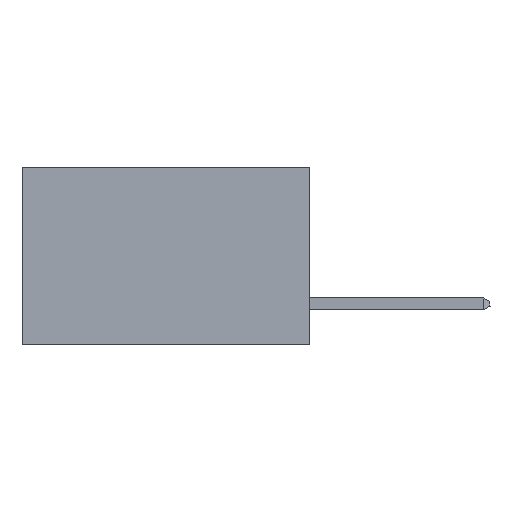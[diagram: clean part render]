
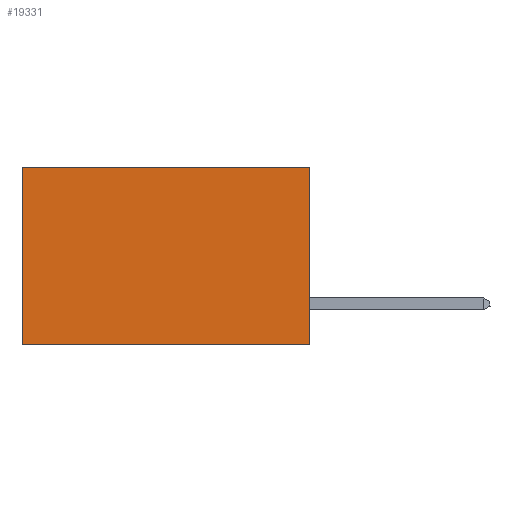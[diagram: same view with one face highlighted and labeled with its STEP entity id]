
A CAD part, left-side view. The second image highlights one B-rep face of the part: STEP entity #19331.
In plain terms, the highlighted planar face has unit normal (-1, 0, 0).
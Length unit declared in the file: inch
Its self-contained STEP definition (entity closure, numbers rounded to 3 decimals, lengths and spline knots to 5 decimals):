
#1119 = VERTEX_POINT ( 'NONE', #47202 ) ;
#1711 = CARTESIAN_POINT ( 'NONE',  ( 0.2875, 0., -0.37 ) ) ;
#5896 = AXIS2_PLACEMENT_3D ( 'NONE', #39786, #47557, #16915 ) ;
#8438 = EDGE_CURVE ( 'NONE', #30630, #1119, #39159, .T. ) ;
#9958 = CARTESIAN_POINT ( 'NONE',  ( 0.2875, 0.6, 0. ) ) ;
#10521 = EDGE_CURVE ( 'NONE', #29294, #42507, #29275, .T. ) ;
#12382 = DIRECTION ( 'NONE',  ( 0., 0., -1. ) ) ;
#14292 = CARTESIAN_POINT ( 'NONE',  ( 0.2875, 0., 0. ) ) ;
#16915 = DIRECTION ( 'NONE',  ( 0., 0., -1. ) ) ;
#17971 = VECTOR ( 'NONE', #47672, 39.37008 ) ;
#18190 = EDGE_CURVE ( 'NONE', #42507, #1119, #22949, .T. ) ;
#19331 = ADVANCED_FACE ( 'NONE', ( #45327 ), #46904, .F. ) ;
#19343 = DIRECTION ( 'NONE',  ( 0., 0., -1. ) ) ;
#22949 = LINE ( 'NONE', #34954, #25308 ) ;
#25308 = VECTOR ( 'NONE', #27547, 39.37008 ) ;
#27218 = CARTESIAN_POINT ( 'NONE',  ( 0.2875, 0., 0. ) ) ;
#27547 = DIRECTION ( 'NONE',  ( 0., 1., 0. ) ) ;
#27829 = ORIENTED_EDGE ( 'NONE', *, *, #30972, .T. ) ;
#29275 = LINE ( 'NONE', #27218, #38107 ) ;
#29294 = VERTEX_POINT ( 'NONE', #14292 ) ;
#30630 = VERTEX_POINT ( 'NONE', #37359 ) ;
#30972 = EDGE_CURVE ( 'NONE', #29294, #30630, #37997, .T. ) ;
#30981 = ORIENTED_EDGE ( 'NONE', *, *, #10521, .F. ) ;
#32502 = ORIENTED_EDGE ( 'NONE', *, *, #8438, .T. ) ;
#34954 = CARTESIAN_POINT ( 'NONE',  ( 0.2875, 0., -0.37 ) ) ;
#36873 = ORIENTED_EDGE ( 'NONE', *, *, #18190, .F. ) ;
#37359 = CARTESIAN_POINT ( 'NONE',  ( 0.2875, 0.6, 0. ) ) ;
#37997 = LINE ( 'NONE', #47501, #17971 ) ;
#38107 = VECTOR ( 'NONE', #19343, 39.37008 ) ;
#39159 = LINE ( 'NONE', #9958, #46220 ) ;
#39786 = CARTESIAN_POINT ( 'NONE',  ( 0.2875, 0., 0. ) ) ;
#42507 = VERTEX_POINT ( 'NONE', #1711 ) ;
#43944 = EDGE_LOOP ( 'NONE', ( #32502, #36873, #30981, #27829 ) ) ;
#45327 = FACE_OUTER_BOUND ( 'NONE', #43944, .T. ) ;
#46220 = VECTOR ( 'NONE', #12382, 39.37008 ) ;
#46904 = PLANE ( 'NONE',  #5896 ) ;
#47202 = CARTESIAN_POINT ( 'NONE',  ( 0.2875, 0.6, -0.37 ) ) ;
#47501 = CARTESIAN_POINT ( 'NONE',  ( 0.2875, 0., 0. ) ) ;
#47557 = DIRECTION ( 'NONE',  ( 1., 0., 0. ) ) ;
#47672 = DIRECTION ( 'NONE',  ( 0., 1., 0. ) ) ;
